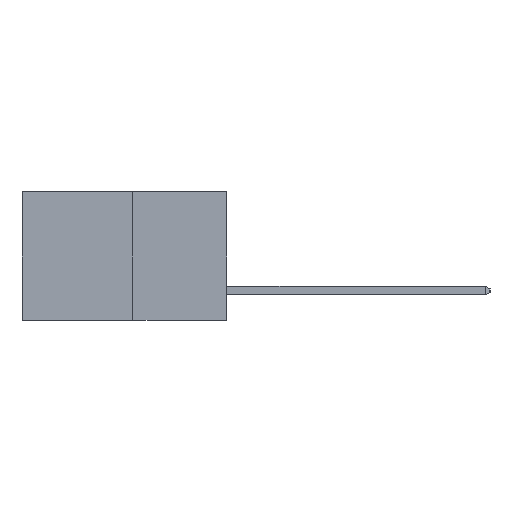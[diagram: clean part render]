
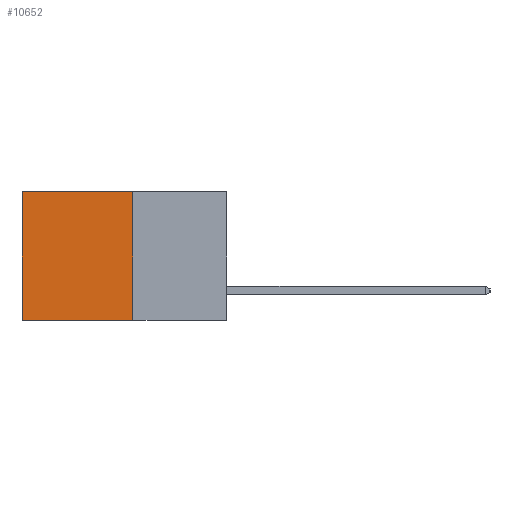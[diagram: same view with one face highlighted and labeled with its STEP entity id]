
A CAD part, left-side view. The second image highlights one B-rep face of the part: STEP entity #10652.
In plain terms, the highlighted planar face has unit normal (-1, 0, 0).
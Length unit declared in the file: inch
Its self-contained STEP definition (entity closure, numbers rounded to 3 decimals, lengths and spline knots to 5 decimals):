
#3229 = EDGE_CURVE ( 'NONE', #8833, #15868, #9765, .T. ) ;
#3781 = VERTEX_POINT ( 'NONE', #17372 ) ;
#3974 = CARTESIAN_POINT ( 'NONE',  ( 0.277, 0.27, -0.37 ) ) ;
#4422 = DIRECTION ( 'NONE',  ( 0., 0., -1. ) ) ;
#5344 = ORIENTED_EDGE ( 'NONE', *, *, #5634, .T. ) ;
#5593 = PLANE ( 'NONE',  #17780 ) ;
#5599 = LINE ( 'NONE', #6806, #18832 ) ;
#5634 = EDGE_CURVE ( 'NONE', #3781, #8833, #5599, .T. ) ;
#5975 = VECTOR ( 'NONE', #6638, 39.37008 ) ;
#6355 = VECTOR ( 'NONE', #10857, 39.37008 ) ;
#6638 = DIRECTION ( 'NONE',  ( 0., 0., -1. ) ) ;
#6806 = CARTESIAN_POINT ( 'NONE',  ( 0.277, 0.27, 0. ) ) ;
#7211 = DIRECTION ( 'NONE',  ( 1., 0., 0. ) ) ;
#7562 = FACE_OUTER_BOUND ( 'NONE', #16799, .T. ) ;
#8430 = DIRECTION ( 'NONE',  ( 0., 1., 0. ) ) ;
#8798 = VECTOR ( 'NONE', #4422, 39.37008 ) ;
#8833 = VERTEX_POINT ( 'NONE', #15196 ) ;
#9765 = LINE ( 'NONE', #14608, #5975 ) ;
#10617 = LINE ( 'NONE', #15674, #6355 ) ;
#10652 = ADVANCED_FACE ( 'NONE', ( #7562 ), #5593, .F. ) ;
#10857 = DIRECTION ( 'NONE',  ( 0., 1., 0. ) ) ;
#11744 = ORIENTED_EDGE ( 'NONE', *, *, #14298, .F. ) ;
#12424 = CARTESIAN_POINT ( 'NONE',  ( 0.277, 0.27, -0.37 ) ) ;
#12707 = EDGE_CURVE ( 'NONE', #14016, #15868, #10617, .T. ) ;
#14014 = LINE ( 'NONE', #12424, #8798 ) ;
#14016 = VERTEX_POINT ( 'NONE', #18715 ) ;
#14274 = ORIENTED_EDGE ( 'NONE', *, *, #3229, .T. ) ;
#14298 = EDGE_CURVE ( 'NONE', #3781, #14016, #14014, .T. ) ;
#14608 = CARTESIAN_POINT ( 'NONE',  ( 0.277, 0.59, -0.37 ) ) ;
#15196 = CARTESIAN_POINT ( 'NONE',  ( 0.277, 0.59, 0. ) ) ;
#15674 = CARTESIAN_POINT ( 'NONE',  ( 0.277, 0.27, -0.37 ) ) ;
#15868 = VERTEX_POINT ( 'NONE', #19569 ) ;
#16721 = ORIENTED_EDGE ( 'NONE', *, *, #12707, .F. ) ;
#16799 = EDGE_LOOP ( 'NONE', ( #14274, #16721, #11744, #5344 ) ) ;
#17372 = CARTESIAN_POINT ( 'NONE',  ( 0.277, 0.27, 0. ) ) ;
#17780 = AXIS2_PLACEMENT_3D ( 'NONE', #3974, #7211, #18367 ) ;
#18367 = DIRECTION ( 'NONE',  ( 0., 0., -1. ) ) ;
#18715 = CARTESIAN_POINT ( 'NONE',  ( 0.277, 0.27, -0.37 ) ) ;
#18832 = VECTOR ( 'NONE', #8430, 39.37008 ) ;
#19569 = CARTESIAN_POINT ( 'NONE',  ( 0.277, 0.59, -0.37 ) ) ;
